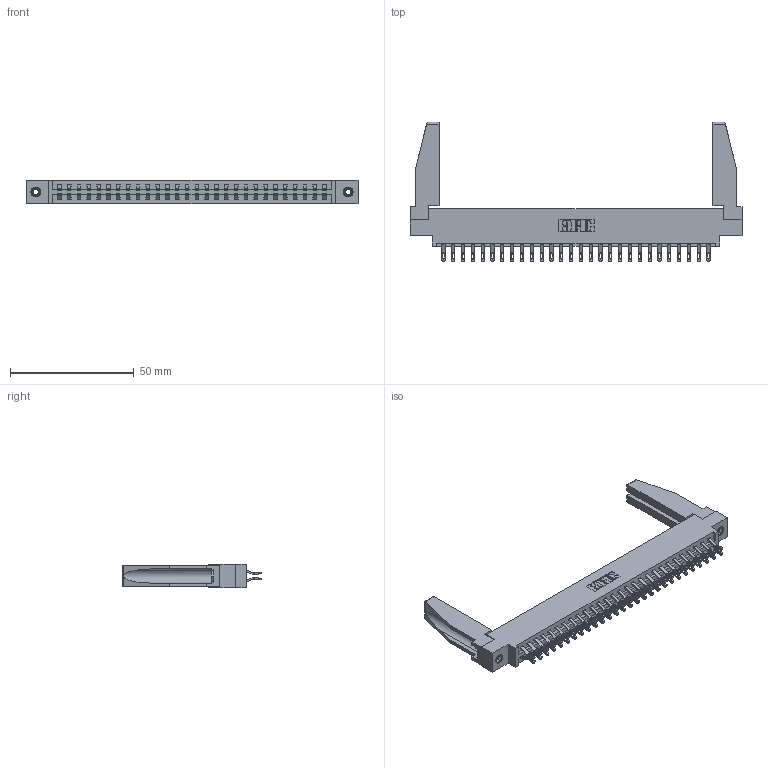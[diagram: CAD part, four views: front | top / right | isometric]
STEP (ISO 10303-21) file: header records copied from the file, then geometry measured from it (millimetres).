
FILE_DESCRIPTION (( 'STEP AP203' ), '1' );
FILE_NAME ('387-056-555-878.STEP', '2019-10-19T07:34:35', ( '' ), ( '' ), 'SwSTEP 2.0', 'SolidWorks 2016', '' );
FILE_SCHEMA (( 'CONFIG_CONTROL_DESIGN' ));
Length unit declared in the file: inch
Products named in the file (5): 337 Part_0.170 Offset - 0.156 Dia-TI; 345-292-001_555 Tail; 345-250-001_345-250-001-102; 307-220-078; 387-056-555-878
Assembly tree (61 placements, depth 2):
  387-056-555-878
    337 Part_0.170 Offset - 0.156 Dia-TI
    345-292-001_555 Tail  x56
    345-250-001_345-250-001-102  x2
    307-220-078  x2
Bounding box: 133.96 x 56.27 x 9.4 mm (x, y, z)
Volume: 17969.6 mm3; surface area: 20214.7 mm2
Topology: 61 solids, 61 shells, 3608 faces, 11237 edges, 7482 vertices
Faces by surface type: plane 2174, cylinder 1418, cone 12, torus 4
Entity records: 26418 total; most frequent: CARTESIAN_POINT 4498, ORIENTED_EDGE 4360, DIRECTION 3828, EDGE_CURVE 2180, LINE 1994, VECTOR 1994, VERTEX_POINT 1448, AXIS2_PLACEMENT_3D 917
